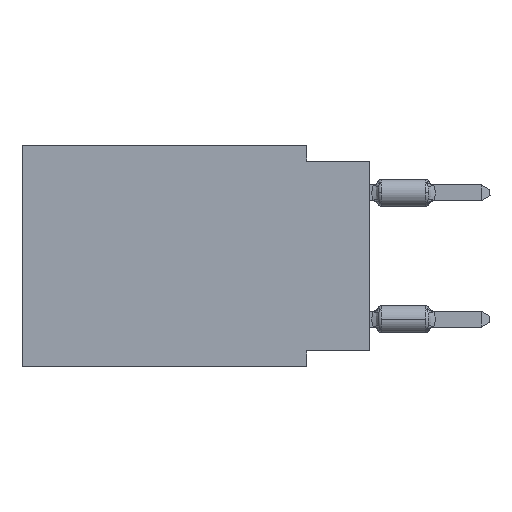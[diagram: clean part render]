
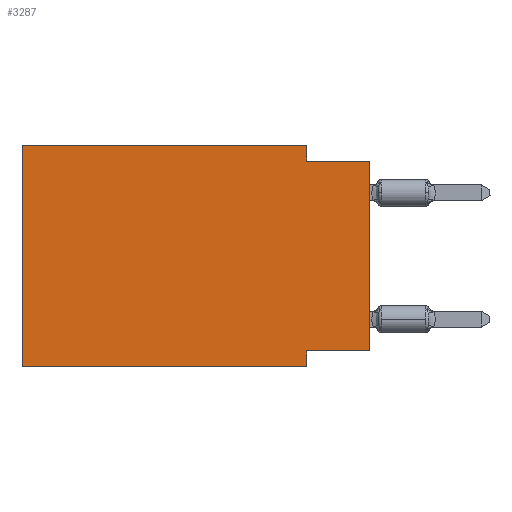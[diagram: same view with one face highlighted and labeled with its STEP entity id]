
A CAD part, left-side view. The second image highlights one B-rep face of the part: STEP entity #3287.
In plain terms, the highlighted planar face has unit normal (-1, 0, 0).
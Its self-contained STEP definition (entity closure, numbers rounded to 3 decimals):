
#552 = VERTEX_POINT ( 'NONE', #16421 ) ;
#1856 = CARTESIAN_POINT ( 'NONE',  ( 0., 2.54, 0. ) ) ;
#2308 = VECTOR ( 'NONE', #15350, 1000. ) ;
#2423 = CARTESIAN_POINT ( 'NONE',  ( 0., 13.97, -8.89 ) ) ;
#3287 = ADVANCED_FACE ( 'NONE', ( #6453 ), #12345, .F. ) ;
#3633 = DIRECTION ( 'NONE',  ( 0., -1., 0. ) ) ;
#3703 = DIRECTION ( 'NONE',  ( 0., -1., 0. ) ) ;
#3925 = CARTESIAN_POINT ( 'NONE',  ( 0., 0., -8.255 ) ) ;
#4983 = ORIENTED_EDGE ( 'NONE', *, *, #12086, .F. ) ;
#5238 = CARTESIAN_POINT ( 'NONE',  ( 0., 0., -0.635 ) ) ;
#5433 = EDGE_CURVE ( 'NONE', #12684, #6081, #8991, .T. ) ;
#5651 = LINE ( 'NONE', #22741, #8786 ) ;
#5870 = VECTOR ( 'NONE', #6096, 1000. ) ;
#5905 = DIRECTION ( 'NONE',  ( 0., 0., 1. ) ) ;
#6014 = AXIS2_PLACEMENT_3D ( 'NONE', #19837, #23412, #14069 ) ;
#6081 = VERTEX_POINT ( 'NONE', #19253 ) ;
#6096 = DIRECTION ( 'NONE',  ( 0., -1., 0. ) ) ;
#6130 = LINE ( 'NONE', #3925, #2308 ) ;
#6453 = FACE_OUTER_BOUND ( 'NONE', #20640, .T. ) ;
#6493 = VERTEX_POINT ( 'NONE', #21298 ) ;
#7110 = CARTESIAN_POINT ( 'NONE',  ( 0., 2.54, 0. ) ) ;
#7206 = CARTESIAN_POINT ( 'NONE',  ( 0., 2.54, -8.89 ) ) ;
#7381 = VECTOR ( 'NONE', #3703, 1000. ) ;
#7657 = ORIENTED_EDGE ( 'NONE', *, *, #11667, .F. ) ;
#7701 = EDGE_CURVE ( 'NONE', #552, #21181, #8171, .T. ) ;
#8055 = CARTESIAN_POINT ( 'NONE',  ( 0., 0., -8.255 ) ) ;
#8058 = LINE ( 'NONE', #2423, #5870 ) ;
#8171 = LINE ( 'NONE', #10243, #24206 ) ;
#8786 = VECTOR ( 'NONE', #5905, 1000. ) ;
#8878 = LINE ( 'NONE', #18571, #7381 ) ;
#8991 = LINE ( 'NONE', #1856, #9932 ) ;
#9354 = DIRECTION ( 'NONE',  ( 0., 0., 1. ) ) ;
#9481 = VERTEX_POINT ( 'NONE', #18592 ) ;
#9932 = VECTOR ( 'NONE', #22000, 1000. ) ;
#10243 = CARTESIAN_POINT ( 'NONE',  ( 0., 2.54, -8.89 ) ) ;
#10750 = LINE ( 'NONE', #12842, #17627 ) ;
#11101 = EDGE_CURVE ( 'NONE', #9481, #12684, #8878, .T. ) ;
#11667 = EDGE_CURVE ( 'NONE', #14556, #552, #6130, .T. ) ;
#11840 = ORIENTED_EDGE ( 'NONE', *, *, #22597, .T. ) ;
#12086 = EDGE_CURVE ( 'NONE', #6081, #23392, #10750, .T. ) ;
#12345 = PLANE ( 'NONE',  #6014 ) ;
#12460 = EDGE_CURVE ( 'NONE', #14556, #23392, #24095, .T. ) ;
#12684 = VERTEX_POINT ( 'NONE', #7110 ) ;
#12842 = CARTESIAN_POINT ( 'NONE',  ( 0., 0., -0.635 ) ) ;
#14069 = DIRECTION ( 'NONE',  ( 0., 0., -1. ) ) ;
#14556 = VERTEX_POINT ( 'NONE', #8055 ) ;
#14802 = ORIENTED_EDGE ( 'NONE', *, *, #7701, .F. ) ;
#15350 = DIRECTION ( 'NONE',  ( 0., 1., 0. ) ) ;
#16421 = CARTESIAN_POINT ( 'NONE',  ( 0., 2.54, -8.255 ) ) ;
#17627 = VECTOR ( 'NONE', #3633, 1000. ) ;
#17636 = DIRECTION ( 'NONE',  ( 0., 0., -1. ) ) ;
#18144 = EDGE_CURVE ( 'NONE', #6493, #9481, #5651, .T. ) ;
#18571 = CARTESIAN_POINT ( 'NONE',  ( 0., 13.97, 0. ) ) ;
#18592 = CARTESIAN_POINT ( 'NONE',  ( 0., 13.97, 0. ) ) ;
#19253 = CARTESIAN_POINT ( 'NONE',  ( 0., 2.54, -0.635 ) ) ;
#19837 = CARTESIAN_POINT ( 'NONE',  ( 0., 13.97, 0. ) ) ;
#20207 = ORIENTED_EDGE ( 'NONE', *, *, #5433, .F. ) ;
#20524 = CARTESIAN_POINT ( 'NONE',  ( 0., 0., 0. ) ) ;
#20640 = EDGE_LOOP ( 'NONE', ( #22568, #4983, #20207, #22577, #22951, #11840, #14802, #7657 ) ) ;
#21161 = VECTOR ( 'NONE', #9354, 1000. ) ;
#21181 = VERTEX_POINT ( 'NONE', #7206 ) ;
#21298 = CARTESIAN_POINT ( 'NONE',  ( 0., 13.97, -8.89 ) ) ;
#22000 = DIRECTION ( 'NONE',  ( 0., 0., -1. ) ) ;
#22568 = ORIENTED_EDGE ( 'NONE', *, *, #12460, .T. ) ;
#22577 = ORIENTED_EDGE ( 'NONE', *, *, #11101, .F. ) ;
#22597 = EDGE_CURVE ( 'NONE', #6493, #21181, #8058, .T. ) ;
#22741 = CARTESIAN_POINT ( 'NONE',  ( 0., 13.97, 0. ) ) ;
#22951 = ORIENTED_EDGE ( 'NONE', *, *, #18144, .F. ) ;
#23392 = VERTEX_POINT ( 'NONE', #5238 ) ;
#23412 = DIRECTION ( 'NONE',  ( 1., 0., 0. ) ) ;
#24095 = LINE ( 'NONE', #20524, #21161 ) ;
#24206 = VECTOR ( 'NONE', #17636, 1000. ) ;
